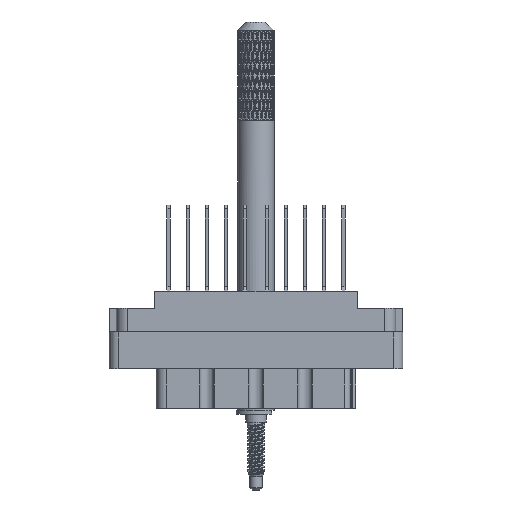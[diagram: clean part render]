
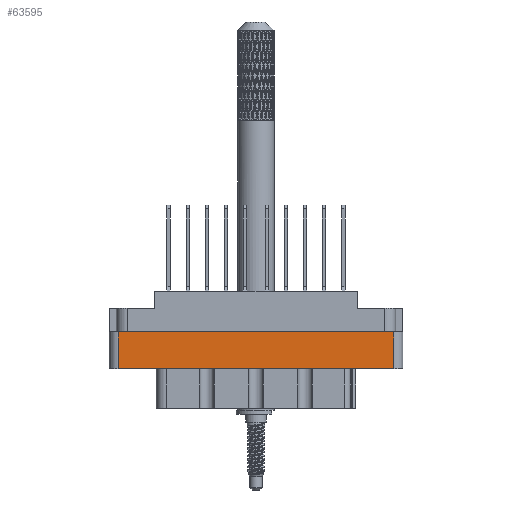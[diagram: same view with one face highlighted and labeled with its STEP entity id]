
A CAD part, front view. The second image highlights one B-rep face of the part: STEP entity #63595.
In plain terms, the highlighted planar face has unit normal (0, -1, 0).
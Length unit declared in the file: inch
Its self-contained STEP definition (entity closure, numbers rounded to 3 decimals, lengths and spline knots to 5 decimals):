
#4807 = VECTOR ( 'NONE', #59559, 39.37008 ) ;
#6582 = DIRECTION ( 'NONE',  ( 0., 0., -1. ) ) ;
#10193 = VERTEX_POINT ( 'NONE', #22300 ) ;
#22300 = CARTESIAN_POINT ( 'NONE',  ( 0.938, -0.438, -0.277 ) ) ;
#22515 = FACE_OUTER_BOUND ( 'NONE', #72261, .T. ) ;
#25853 = CARTESIAN_POINT ( 'NONE',  ( 0.938, -0.438, -0.529 ) ) ;
#26357 = EDGE_CURVE ( 'NONE', #36972, #48414, #49483, .T. ) ;
#31437 = CARTESIAN_POINT ( 'NONE',  ( 0., -0.438, -0.277 ) ) ;
#33233 = DIRECTION ( 'NONE',  ( 0., 0., -1. ) ) ;
#35342 = EDGE_CURVE ( 'NONE', #64007, #10193, #57442, .T. ) ;
#36806 = VECTOR ( 'NONE', #41305, 39.37008 ) ;
#36972 = VERTEX_POINT ( 'NONE', #25853 ) ;
#37378 = AXIS2_PLACEMENT_3D ( 'NONE', #39741, #104635, #6582 ) ;
#37457 = VECTOR ( 'NONE', #33233, 39.37008 ) ;
#39741 = CARTESIAN_POINT ( 'NONE',  ( -1., -0.438, -0.798 ) ) ;
#41305 = DIRECTION ( 'NONE',  ( -1., 0., 0. ) ) ;
#48414 = VERTEX_POINT ( 'NONE', #100889 ) ;
#48465 = CARTESIAN_POINT ( 'NONE',  ( -0.938, -0.438, -0.798 ) ) ;
#48837 = LINE ( 'NONE', #50788, #4807 ) ;
#49483 = LINE ( 'NONE', #81825, #36806 ) ;
#50788 = CARTESIAN_POINT ( 'NONE',  ( 0.938, -0.438, -0.798 ) ) ;
#52520 = EDGE_CURVE ( 'NONE', #64007, #48414, #99310, .T. ) ;
#57442 = LINE ( 'NONE', #31437, #92779 ) ;
#59559 = DIRECTION ( 'NONE',  ( 0., 0., 1. ) ) ;
#63595 = ADVANCED_FACE ( 'NONE', ( #22515 ), #79929, .T. ) ;
#64007 = VERTEX_POINT ( 'NONE', #102802 ) ;
#64936 = ORIENTED_EDGE ( 'NONE', *, *, #35342, .F. ) ;
#72261 = EDGE_LOOP ( 'NONE', ( #64936, #103014, #93001, #92734 ) ) ;
#79929 = PLANE ( 'NONE',  #37378 ) ;
#81825 = CARTESIAN_POINT ( 'NONE',  ( 0., -0.438, -0.529 ) ) ;
#87596 = DIRECTION ( 'NONE',  ( 1., 0., 0. ) ) ;
#92734 = ORIENTED_EDGE ( 'NONE', *, *, #101526, .T. ) ;
#92779 = VECTOR ( 'NONE', #87596, 39.37008 ) ;
#93001 = ORIENTED_EDGE ( 'NONE', *, *, #26357, .F. ) ;
#99310 = LINE ( 'NONE', #48465, #37457 ) ;
#100889 = CARTESIAN_POINT ( 'NONE',  ( -0.938, -0.438, -0.529 ) ) ;
#101526 = EDGE_CURVE ( 'NONE', #36972, #10193, #48837, .T. ) ;
#102802 = CARTESIAN_POINT ( 'NONE',  ( -0.938, -0.438, -0.277 ) ) ;
#103014 = ORIENTED_EDGE ( 'NONE', *, *, #52520, .T. ) ;
#104635 = DIRECTION ( 'NONE',  ( 0., -1., 0. ) ) ;
